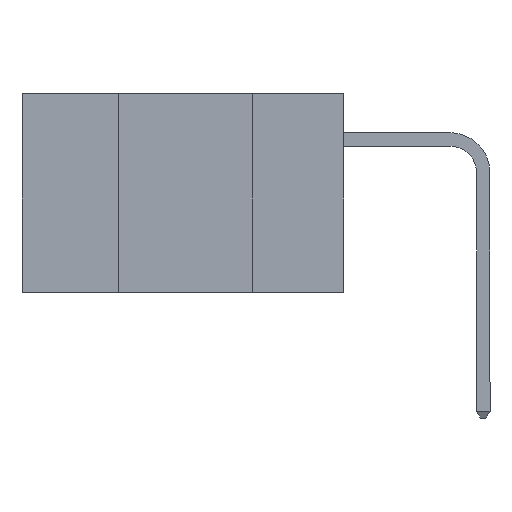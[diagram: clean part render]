
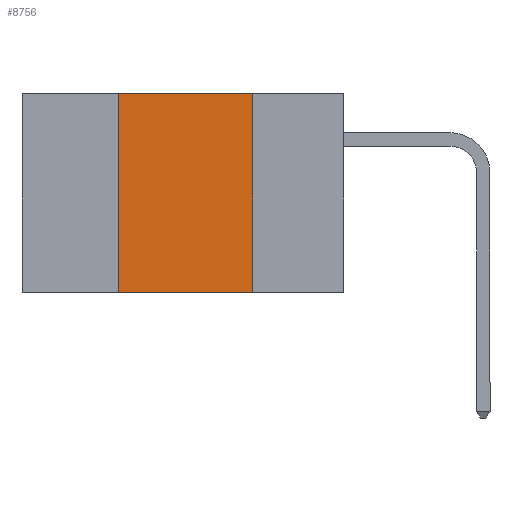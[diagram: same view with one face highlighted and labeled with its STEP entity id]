
A CAD part, left-side view. The second image highlights one B-rep face of the part: STEP entity #8756.
In plain terms, the highlighted planar face has unit normal (-1, 0, 0).
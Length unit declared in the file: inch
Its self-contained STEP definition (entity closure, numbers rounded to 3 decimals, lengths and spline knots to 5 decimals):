
#5 = EDGE_CURVE ( 'NONE', #8412, #9539, #5976, .T. ) ;
#382 = DIRECTION ( 'NONE',  ( 0., 0., -1. ) ) ;
#807 = EDGE_CURVE ( 'NONE', #6569, #4831, #9345, .T. ) ;
#1008 = VECTOR ( 'NONE', #1790, 39.37008 ) ;
#1018 = PLANE ( 'NONE',  #11835 ) ;
#1790 = DIRECTION ( 'NONE',  ( 0., -1., 0. ) ) ;
#2551 = ORIENTED_EDGE ( 'NONE', *, *, #807, .F. ) ;
#2596 = ORIENTED_EDGE ( 'NONE', *, *, #4733, .F. ) ;
#2623 = CARTESIAN_POINT ( 'NONE',  ( 0., 0.6, 0. ) ) ;
#2626 = ORIENTED_EDGE ( 'NONE', *, *, #5, .F. ) ;
#2657 = ORIENTED_EDGE ( 'NONE', *, *, #12348, .T. ) ;
#3102 = VECTOR ( 'NONE', #13304, 39.37008 ) ;
#4733 = EDGE_CURVE ( 'NONE', #9539, #6569, #11111, .T. ) ;
#4831 = VERTEX_POINT ( 'NONE', #9580 ) ;
#5452 = DIRECTION ( 'NONE',  ( 1., 0., 0. ) ) ;
#5976 = LINE ( 'NONE', #13432, #3102 ) ;
#6560 = FACE_OUTER_BOUND ( 'NONE', #8245, .T. ) ;
#6569 = VERTEX_POINT ( 'NONE', #9873 ) ;
#6574 = DIRECTION ( 'NONE',  ( 0., -1., 0. ) ) ;
#6994 = CARTESIAN_POINT ( 'NONE',  ( 0., 0.42, 0. ) ) ;
#8245 = EDGE_LOOP ( 'NONE', ( #2551, #2596, #2626, #2657 ) ) ;
#8403 = VECTOR ( 'NONE', #6574, 39.37008 ) ;
#8412 = VERTEX_POINT ( 'NONE', #10060 ) ;
#8756 = ADVANCED_FACE ( 'NONE', ( #6560 ), #1018, .F. ) ;
#9240 = CARTESIAN_POINT ( 'NONE',  ( 0., 0.6, -0.37 ) ) ;
#9309 = CARTESIAN_POINT ( 'NONE',  ( 0., 0.17, 0. ) ) ;
#9345 = LINE ( 'NONE', #9309, #11961 ) ;
#9539 = VERTEX_POINT ( 'NONE', #6994 ) ;
#9564 = CARTESIAN_POINT ( 'NONE',  ( 0., 0.6, 0. ) ) ;
#9580 = CARTESIAN_POINT ( 'NONE',  ( 0., 0.17, -0.37 ) ) ;
#9873 = CARTESIAN_POINT ( 'NONE',  ( 0., 0.17, 0. ) ) ;
#10060 = CARTESIAN_POINT ( 'NONE',  ( 0., 0.42, -0.37 ) ) ;
#11111 = LINE ( 'NONE', #2623, #8403 ) ;
#11835 = AXIS2_PLACEMENT_3D ( 'NONE', #9564, #5452, #12547 ) ;
#11853 = LINE ( 'NONE', #9240, #1008 ) ;
#11961 = VECTOR ( 'NONE', #382, 39.37008 ) ;
#12348 = EDGE_CURVE ( 'NONE', #8412, #4831, #11853, .T. ) ;
#12547 = DIRECTION ( 'NONE',  ( 0., 0., -1. ) ) ;
#13304 = DIRECTION ( 'NONE',  ( 0., 0., 1. ) ) ;
#13432 = CARTESIAN_POINT ( 'NONE',  ( 0., 0.42, 0. ) ) ;
